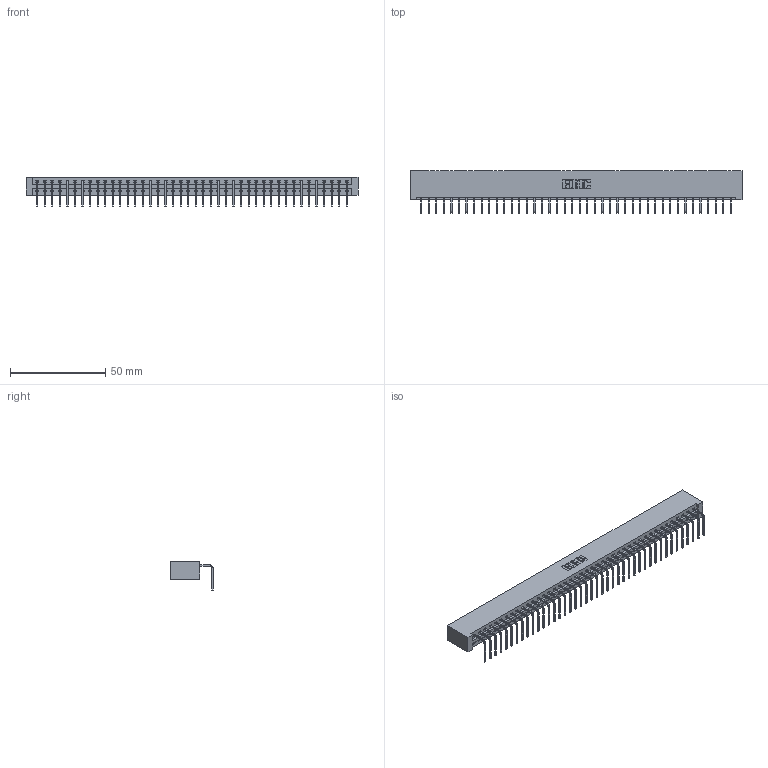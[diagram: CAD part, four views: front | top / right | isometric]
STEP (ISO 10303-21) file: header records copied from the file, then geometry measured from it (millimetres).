
FILE_DESCRIPTION (( 'STEP AP203' ), '1' );
FILE_NAME ('387-042-558-101.STEP', '2019-10-07T21:45:57', ( '' ), ( '' ), 'SwSTEP 2.0', 'SolidWorks 2016', '' );
FILE_SCHEMA (( 'CONFIG_CONTROL_DESIGN' ));
Length unit declared in the file: inch
Products named in the file (3): 345-292-001_558 Tail - 2; 387-042-558-101; 337 Part_No Mounting Lugs
Assembly tree (43 placements, depth 2):
  387-042-558-101
    337 Part_No Mounting Lugs
    345-292-001_558 Tail - 2  x42
Bounding box: 174.29 x 22.17 x 15.37 mm (x, y, z)
Volume: 18993.7 mm3; surface area: 20468.3 mm2
Topology: 43 solids, 43 shells, 2794 faces, 8435 edges, 5566 vertices
Faces by surface type: plane 2082, cylinder 712
Entity records: 31027 total; most frequent: CARTESIAN_POINT 5412, ORIENTED_EDGE 5390, DIRECTION 4547, EDGE_CURVE 2695, LINE 2575, VECTOR 2575, VERTEX_POINT 1794, AXIS2_PLACEMENT_3D 986
